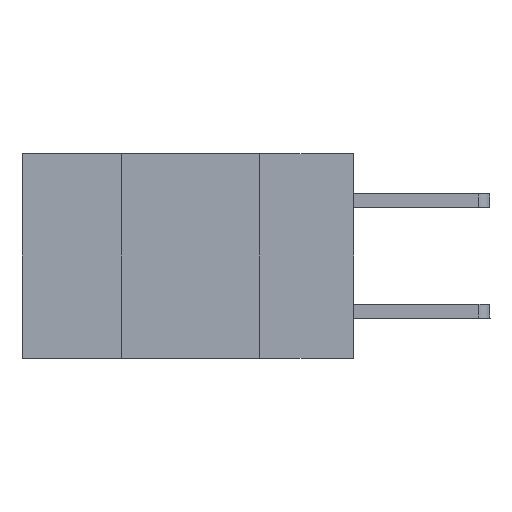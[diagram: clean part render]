
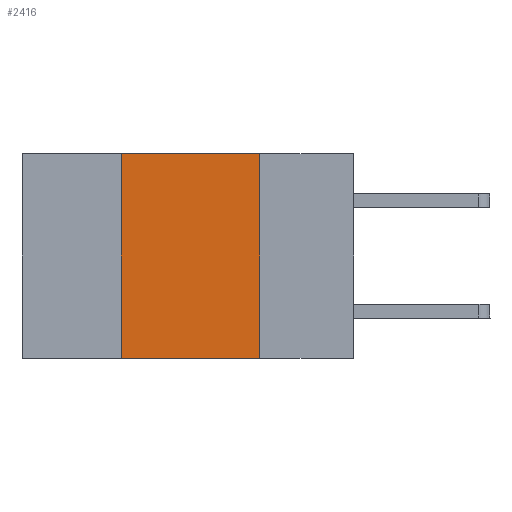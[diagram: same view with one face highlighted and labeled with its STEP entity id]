
A CAD part, left-side view. The second image highlights one B-rep face of the part: STEP entity #2416.
In plain terms, the highlighted planar face has unit normal (-1, 0, 0).
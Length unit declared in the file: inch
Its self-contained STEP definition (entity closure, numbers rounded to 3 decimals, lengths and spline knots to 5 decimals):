
#30 = CARTESIAN_POINT ( 'NONE',  ( 0., 0.42, 0. ) ) ;
#147 = VERTEX_POINT ( 'NONE', #216 ) ;
#216 = CARTESIAN_POINT ( 'NONE',  ( 0., 0.17, -0.37 ) ) ;
#492 = DIRECTION ( 'NONE',  ( 0., -1., 0. ) ) ;
#729 = ORIENTED_EDGE ( 'NONE', *, *, #8065, .T. ) ;
#1077 = FACE_OUTER_BOUND ( 'NONE', #3141, .T. ) ;
#1407 = VERTEX_POINT ( 'NONE', #30 ) ;
#1748 = VECTOR ( 'NONE', #12031, 39.37008 ) ;
#2023 = DIRECTION ( 'NONE',  ( 1., 0., 0. ) ) ;
#2164 = PLANE ( 'NONE',  #3529 ) ;
#2308 = EDGE_CURVE ( 'NONE', #1407, #12453, #2315, .T. ) ;
#2315 = LINE ( 'NONE', #6424, #6696 ) ;
#2416 = ADVANCED_FACE ( 'NONE', ( #1077 ), #2164, .F. ) ;
#3141 = EDGE_LOOP ( 'NONE', ( #9812, #12466, #7996, #729 ) ) ;
#3285 = CARTESIAN_POINT ( 'NONE',  ( 0., 0.6, 0. ) ) ;
#3361 = DIRECTION ( 'NONE',  ( 0., -1., 0. ) ) ;
#3529 = AXIS2_PLACEMENT_3D ( 'NONE', #3285, #2023, #13037 ) ;
#3639 = DIRECTION ( 'NONE',  ( 0., 0., -1. ) ) ;
#4794 = LINE ( 'NONE', #6761, #5348 ) ;
#5348 = VECTOR ( 'NONE', #3639, 39.37008 ) ;
#6424 = CARTESIAN_POINT ( 'NONE',  ( 0., 0.6, 0. ) ) ;
#6696 = VECTOR ( 'NONE', #3361, 39.37008 ) ;
#6761 = CARTESIAN_POINT ( 'NONE',  ( 0., 0.17, 0. ) ) ;
#7321 = CARTESIAN_POINT ( 'NONE',  ( 0., 0.17, 0. ) ) ;
#7546 = LINE ( 'NONE', #7691, #1748 ) ;
#7691 = CARTESIAN_POINT ( 'NONE',  ( 0., 0.42, 0. ) ) ;
#7891 = CARTESIAN_POINT ( 'NONE',  ( 0., 0.6, -0.37 ) ) ;
#7952 = CARTESIAN_POINT ( 'NONE',  ( 0., 0.42, -0.37 ) ) ;
#7996 = ORIENTED_EDGE ( 'NONE', *, *, #10843, .F. ) ;
#8065 = EDGE_CURVE ( 'NONE', #8828, #147, #13520, .T. ) ;
#8176 = EDGE_CURVE ( 'NONE', #12453, #147, #4794, .T. ) ;
#8828 = VERTEX_POINT ( 'NONE', #7952 ) ;
#9812 = ORIENTED_EDGE ( 'NONE', *, *, #8176, .F. ) ;
#10270 = VECTOR ( 'NONE', #492, 39.37008 ) ;
#10843 = EDGE_CURVE ( 'NONE', #8828, #1407, #7546, .T. ) ;
#12031 = DIRECTION ( 'NONE',  ( 0., 0., 1. ) ) ;
#12453 = VERTEX_POINT ( 'NONE', #7321 ) ;
#12466 = ORIENTED_EDGE ( 'NONE', *, *, #2308, .F. ) ;
#13037 = DIRECTION ( 'NONE',  ( 0., 0., -1. ) ) ;
#13520 = LINE ( 'NONE', #7891, #10270 ) ;
